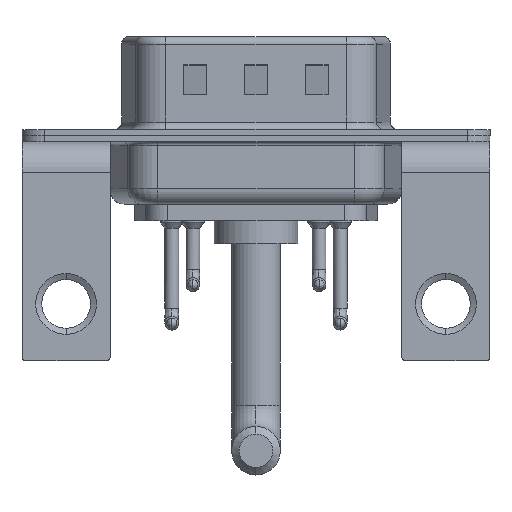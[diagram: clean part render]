
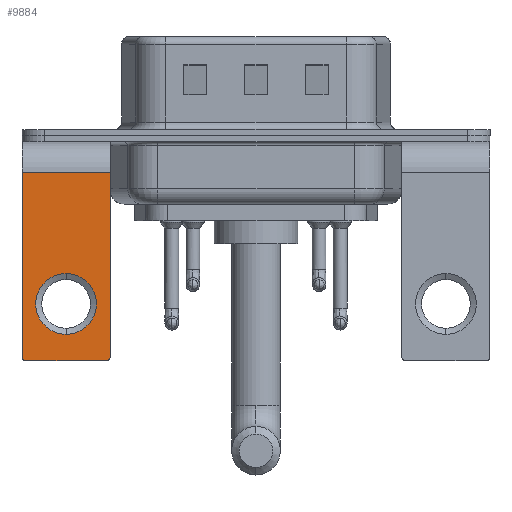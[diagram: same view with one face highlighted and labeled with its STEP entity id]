
A CAD part, front view. The second image highlights one B-rep face of the part: STEP entity #9884.
In plain terms, the highlighted planar face has unit normal (0, -1, 0).
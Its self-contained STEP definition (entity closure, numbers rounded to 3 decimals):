
#69 = CARTESIAN_POINT ( 'NONE',  ( 2.65, -6.25, -14.55 ) ) ;
#1749 = ORIENTED_EDGE ( 'NONE', *, *, #13260, .T. ) ;
#2347 = EDGE_CURVE ( 'NONE', #4840, #14018, #12591, .T. ) ;
#2893 = AXIS2_PLACEMENT_3D ( 'NONE', #10066, #14578, #16201 ) ;
#3064 = EDGE_CURVE ( 'NONE', #3464, #5583, #5661, .T. ) ;
#3375 = CARTESIAN_POINT ( 'NONE',  ( -2.9, -6.25, -2.4 ) ) ;
#3464 = VERTEX_POINT ( 'NONE', #17533 ) ;
#3639 = CIRCLE ( 'NONE', #11834, 0.25 ) ;
#4840 = VERTEX_POINT ( 'NONE', #11858 ) ;
#5211 = EDGE_CURVE ( 'NONE', #7818, #14018, #10592, .T. ) ;
#5290 = CARTESIAN_POINT ( 'NONE',  ( -2.65, -6.25, -14.8 ) ) ;
#5305 = ORIENTED_EDGE ( 'NONE', *, *, #3064, .T. ) ;
#5506 = CARTESIAN_POINT ( 'NONE',  ( 2.9, -6.25, -2.4 ) ) ;
#5577 = CARTESIAN_POINT ( 'NONE',  ( 2.9, -6.25, -14.8 ) ) ;
#5583 = VERTEX_POINT ( 'NONE', #14270 ) ;
#5661 = LINE ( 'NONE', #18079, #14903 ) ;
#5733 = DIRECTION ( 'NONE',  ( 0., -1., 0. ) ) ;
#5826 = DIRECTION ( 'NONE',  ( 0., 0., 1. ) ) ;
#6239 = CARTESIAN_POINT ( 'NONE',  ( 2.65, -6.25, -14.8 ) ) ;
#6433 = CIRCLE ( 'NONE', #16012, 2. ) ;
#6634 = ORIENTED_EDGE ( 'NONE', *, *, #7815, .T. ) ;
#6703 = VERTEX_POINT ( 'NONE', #10456 ) ;
#7151 = DIRECTION ( 'NONE',  ( 0., 0., -1. ) ) ;
#7263 = LINE ( 'NONE', #5506, #9769 ) ;
#7815 = EDGE_CURVE ( 'NONE', #16401, #6703, #6433, .T. ) ;
#7818 = VERTEX_POINT ( 'NONE', #6239 ) ;
#8532 = FACE_OUTER_BOUND ( 'NONE', #17306, .T. ) ;
#8829 = CARTESIAN_POINT ( 'NONE',  ( 0., -6.25, -9.07 ) ) ;
#9769 = VECTOR ( 'NONE', #7151, 1000. ) ;
#9875 = FACE_BOUND ( 'NONE', #16148, .T. ) ;
#9884 = ADVANCED_FACE ( 'NONE', ( #9875, #8532 ), #13146, .F. ) ;
#10066 = CARTESIAN_POINT ( 'NONE',  ( 2.9, -6.25, -2.4 ) ) ;
#10100 = EDGE_CURVE ( 'NONE', #6703, #16401, #19609, .T. ) ;
#10280 = DIRECTION ( 'NONE',  ( -1., 0., 0. ) ) ;
#10293 = AXIS2_PLACEMENT_3D ( 'NONE', #16892, #5733, #5826 ) ;
#10371 = CARTESIAN_POINT ( 'NONE',  ( 0., -6.25, -11.07 ) ) ;
#10456 = CARTESIAN_POINT ( 'NONE',  ( 0., -6.25, -13.07 ) ) ;
#10592 = LINE ( 'NONE', #5577, #14784 ) ;
#10757 = AXIS2_PLACEMENT_3D ( 'NONE', #10371, #14981, #12225 ) ;
#10805 = VECTOR ( 'NONE', #19070, 1000. ) ;
#11515 = ORIENTED_EDGE ( 'NONE', *, *, #10100, .T. ) ;
#11834 = AXIS2_PLACEMENT_3D ( 'NONE', #69, #14025, #15362 ) ;
#11858 = CARTESIAN_POINT ( 'NONE',  ( -2.9, -6.25, -14.55 ) ) ;
#12199 = DIRECTION ( 'NONE',  ( 0., 1., 0. ) ) ;
#12225 = DIRECTION ( 'NONE',  ( 0., 0., 1. ) ) ;
#12591 = CIRCLE ( 'NONE', #10293, 0.25 ) ;
#13104 = LINE ( 'NONE', #3375, #10805 ) ;
#13146 = PLANE ( 'NONE',  #2893 ) ;
#13260 = EDGE_CURVE ( 'NONE', #5583, #4840, #13104, .T. ) ;
#13924 = DIRECTION ( 'NONE',  ( 0., 0., 1. ) ) ;
#14018 = VERTEX_POINT ( 'NONE', #5290 ) ;
#14025 = DIRECTION ( 'NONE',  ( 0., -1., 0. ) ) ;
#14270 = CARTESIAN_POINT ( 'NONE',  ( -2.9, -6.25, -2.4 ) ) ;
#14578 = DIRECTION ( 'NONE',  ( 0., 1., 0. ) ) ;
#14784 = VECTOR ( 'NONE', #18185, 1000. ) ;
#14903 = VECTOR ( 'NONE', #10280, 1000. ) ;
#14981 = DIRECTION ( 'NONE',  ( 0., 1., 0. ) ) ;
#15036 = CARTESIAN_POINT ( 'NONE',  ( 2.9, -6.25, -14.55 ) ) ;
#15162 = CARTESIAN_POINT ( 'NONE',  ( 0., -6.25, -11.07 ) ) ;
#15362 = DIRECTION ( 'NONE',  ( 0., 0., 1. ) ) ;
#16012 = AXIS2_PLACEMENT_3D ( 'NONE', #15162, #12199, #13924 ) ;
#16148 = EDGE_LOOP ( 'NONE', ( #11515, #6634 ) ) ;
#16201 = DIRECTION ( 'NONE',  ( 0., 0., 1. ) ) ;
#16207 = ORIENTED_EDGE ( 'NONE', *, *, #2347, .T. ) ;
#16401 = VERTEX_POINT ( 'NONE', #8829 ) ;
#16892 = CARTESIAN_POINT ( 'NONE',  ( -2.65, -6.25, -14.55 ) ) ;
#17306 = EDGE_LOOP ( 'NONE', ( #1749, #16207, #19956, #19713, #17489, #5305 ) ) ;
#17489 = ORIENTED_EDGE ( 'NONE', *, *, #20101, .F. ) ;
#17533 = CARTESIAN_POINT ( 'NONE',  ( 2.9, -6.25, -2.4 ) ) ;
#18079 = CARTESIAN_POINT ( 'NONE',  ( 2.9, -6.25, -2.4 ) ) ;
#18185 = DIRECTION ( 'NONE',  ( -1., 0., 0. ) ) ;
#18372 = EDGE_CURVE ( 'NONE', #7818, #18724, #3639, .T. ) ;
#18724 = VERTEX_POINT ( 'NONE', #15036 ) ;
#19070 = DIRECTION ( 'NONE',  ( 0., 0., -1. ) ) ;
#19609 = CIRCLE ( 'NONE', #10757, 2. ) ;
#19713 = ORIENTED_EDGE ( 'NONE', *, *, #18372, .T. ) ;
#19956 = ORIENTED_EDGE ( 'NONE', *, *, #5211, .F. ) ;
#20101 = EDGE_CURVE ( 'NONE', #3464, #18724, #7263, .T. ) ;
